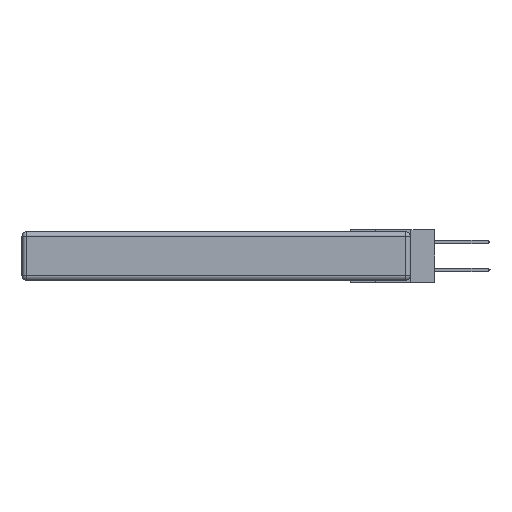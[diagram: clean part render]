
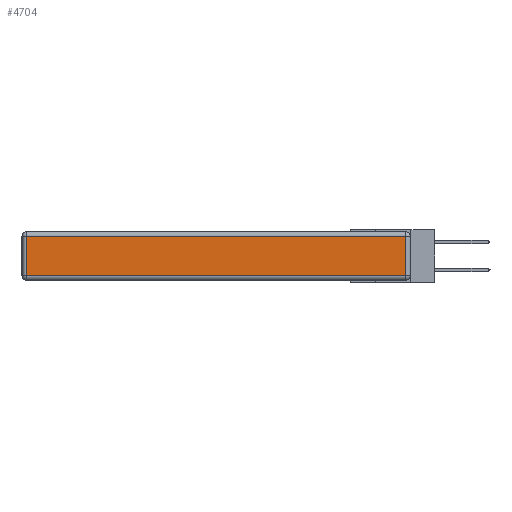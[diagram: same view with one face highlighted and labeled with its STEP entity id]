
A CAD part, left-side view. The second image highlights one B-rep face of the part: STEP entity #4704.
In plain terms, the highlighted planar face has unit normal (-1, 0, 0).
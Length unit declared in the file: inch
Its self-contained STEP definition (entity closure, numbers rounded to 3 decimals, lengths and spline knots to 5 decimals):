
#685 = DIRECTION ( 'NONE',  ( 0., -1., 0. ) ) ;
#753 = CARTESIAN_POINT ( 'NONE',  ( 0., 2.72, -0.03 ) ) ;
#1812 = ORIENTED_EDGE ( 'NONE', *, *, #20207, .T. ) ;
#2170 = ORIENTED_EDGE ( 'NONE', *, *, #4103, .T. ) ;
#2510 = EDGE_CURVE ( 'NONE', #7059, #18971, #19301, .T. ) ;
#3142 = AXIS2_PLACEMENT_3D ( 'NONE', #6140, #20908, #9822 ) ;
#3611 = DIRECTION ( 'NONE',  ( 0., 0., 1. ) ) ;
#4030 = VECTOR ( 'NONE', #19598, 39.37008 ) ;
#4103 = EDGE_CURVE ( 'NONE', #9930, #12065, #8832, .T. ) ;
#4566 = LINE ( 'NONE', #19396, #18328 ) ;
#4704 = ADVANCED_FACE ( 'NONE', ( #14230 ), #17132, .T. ) ;
#6140 = CARTESIAN_POINT ( 'NONE',  ( 0., 0., -0.343 ) ) ;
#6306 = LINE ( 'NONE', #18863, #4030 ) ;
#7059 = VERTEX_POINT ( 'NONE', #753 ) ;
#7205 = EDGE_LOOP ( 'NONE', ( #18600, #2170, #1812, #21404 ) ) ;
#7338 = DIRECTION ( 'NONE',  ( 0., 0., -1. ) ) ;
#7562 = CARTESIAN_POINT ( 'NONE',  ( 0., 2.72, -0.313 ) ) ;
#8259 = VECTOR ( 'NONE', #3611, 39.37008 ) ;
#8832 = LINE ( 'NONE', #16108, #8259 ) ;
#9822 = DIRECTION ( 'NONE',  ( 0., 0., 1. ) ) ;
#9930 = VERTEX_POINT ( 'NONE', #13563 ) ;
#12065 = VERTEX_POINT ( 'NONE', #20536 ) ;
#13226 = VECTOR ( 'NONE', #7338, 39.37008 ) ;
#13563 = CARTESIAN_POINT ( 'NONE',  ( 0., 0.03, -0.313 ) ) ;
#14023 = EDGE_CURVE ( 'NONE', #18971, #9930, #4566, .T. ) ;
#14230 = FACE_OUTER_BOUND ( 'NONE', #7205, .T. ) ;
#14790 = CARTESIAN_POINT ( 'NONE',  ( 0., 2.72, -0.343 ) ) ;
#16108 = CARTESIAN_POINT ( 'NONE',  ( 0., 0.03, -0.343 ) ) ;
#17132 = PLANE ( 'NONE',  #3142 ) ;
#18328 = VECTOR ( 'NONE', #685, 39.37008 ) ;
#18600 = ORIENTED_EDGE ( 'NONE', *, *, #14023, .T. ) ;
#18863 = CARTESIAN_POINT ( 'NONE',  ( 0., 2.75, -0.03 ) ) ;
#18971 = VERTEX_POINT ( 'NONE', #7562 ) ;
#19301 = LINE ( 'NONE', #14790, #13226 ) ;
#19396 = CARTESIAN_POINT ( 'NONE',  ( 0., 0., -0.313 ) ) ;
#19598 = DIRECTION ( 'NONE',  ( 0., 1., 0. ) ) ;
#20207 = EDGE_CURVE ( 'NONE', #12065, #7059, #6306, .T. ) ;
#20536 = CARTESIAN_POINT ( 'NONE',  ( 0., 0.03, -0.03 ) ) ;
#20908 = DIRECTION ( 'NONE',  ( -1., 0., 0. ) ) ;
#21404 = ORIENTED_EDGE ( 'NONE', *, *, #2510, .T. ) ;
